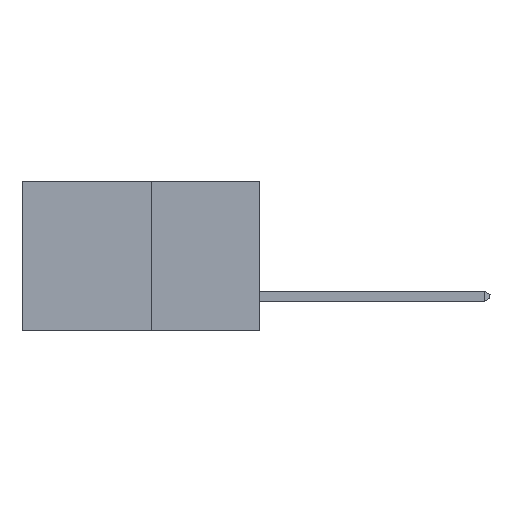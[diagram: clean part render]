
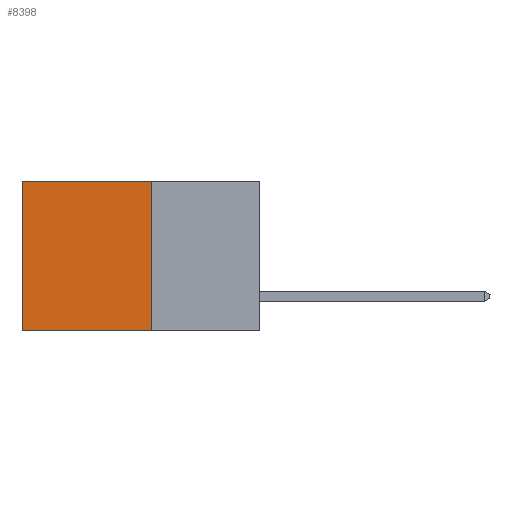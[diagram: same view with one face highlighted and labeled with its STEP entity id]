
A CAD part, left-side view. The second image highlights one B-rep face of the part: STEP entity #8398.
In plain terms, the highlighted planar face has unit normal (-1, 0, 0).
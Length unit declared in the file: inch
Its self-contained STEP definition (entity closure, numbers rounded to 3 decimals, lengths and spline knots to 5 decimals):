
#73 = CARTESIAN_POINT ( 'NONE',  ( 0.277, 0.27, -0.37 ) ) ;
#343 = VERTEX_POINT ( 'NONE', #1925 ) ;
#473 = EDGE_CURVE ( 'NONE', #775, #343, #7606, .T. ) ;
#524 = ORIENTED_EDGE ( 'NONE', *, *, #1815, .T. ) ;
#775 = VERTEX_POINT ( 'NONE', #5371 ) ;
#1044 = CARTESIAN_POINT ( 'NONE',  ( 0.277, 0.27, -0.37 ) ) ;
#1286 = CARTESIAN_POINT ( 'NONE',  ( 0.277, 0.27, 0. ) ) ;
#1346 = DIRECTION ( 'NONE',  ( 0., 1., 0. ) ) ;
#1511 = PLANE ( 'NONE',  #5426 ) ;
#1632 = FACE_OUTER_BOUND ( 'NONE', #5897, .T. ) ;
#1668 = CARTESIAN_POINT ( 'NONE',  ( 0.277, 0.27, 0. ) ) ;
#1709 = EDGE_CURVE ( 'NONE', #2169, #1881, #8880, .T. ) ;
#1815 = EDGE_CURVE ( 'NONE', #1881, #343, #3038, .T. ) ;
#1881 = VERTEX_POINT ( 'NONE', #7770 ) ;
#1925 = CARTESIAN_POINT ( 'NONE',  ( 0.277, 0.59, -0.37 ) ) ;
#2120 = VECTOR ( 'NONE', #5875, 39.37008 ) ;
#2169 = VERTEX_POINT ( 'NONE', #1668 ) ;
#2221 = DIRECTION ( 'NONE',  ( 1., 0., 0. ) ) ;
#2466 = VECTOR ( 'NONE', #4526, 39.37008 ) ;
#3038 = LINE ( 'NONE', #5803, #8270 ) ;
#3339 = EDGE_CURVE ( 'NONE', #2169, #775, #5928, .T. ) ;
#3911 = VECTOR ( 'NONE', #1346, 39.37008 ) ;
#4526 = DIRECTION ( 'NONE',  ( 0., 0., -1. ) ) ;
#4593 = CARTESIAN_POINT ( 'NONE',  ( 0.277, 0.27, -0.37 ) ) ;
#5054 = ORIENTED_EDGE ( 'NONE', *, *, #1709, .T. ) ;
#5371 = CARTESIAN_POINT ( 'NONE',  ( 0.277, 0.27, -0.37 ) ) ;
#5426 = AXIS2_PLACEMENT_3D ( 'NONE', #73, #2221, #7046 ) ;
#5803 = CARTESIAN_POINT ( 'NONE',  ( 0.277, 0.59, -0.37 ) ) ;
#5875 = DIRECTION ( 'NONE',  ( 0., 1., 0. ) ) ;
#5897 = EDGE_LOOP ( 'NONE', ( #524, #7717, #6029, #5054 ) ) ;
#5928 = LINE ( 'NONE', #4593, #2466 ) ;
#6029 = ORIENTED_EDGE ( 'NONE', *, *, #3339, .F. ) ;
#6174 = DIRECTION ( 'NONE',  ( 0., 0., -1. ) ) ;
#7046 = DIRECTION ( 'NONE',  ( 0., 0., -1. ) ) ;
#7606 = LINE ( 'NONE', #1044, #2120 ) ;
#7717 = ORIENTED_EDGE ( 'NONE', *, *, #473, .F. ) ;
#7770 = CARTESIAN_POINT ( 'NONE',  ( 0.277, 0.59, 0. ) ) ;
#8270 = VECTOR ( 'NONE', #6174, 39.37008 ) ;
#8398 = ADVANCED_FACE ( 'NONE', ( #1632 ), #1511, .F. ) ;
#8880 = LINE ( 'NONE', #1286, #3911 ) ;
